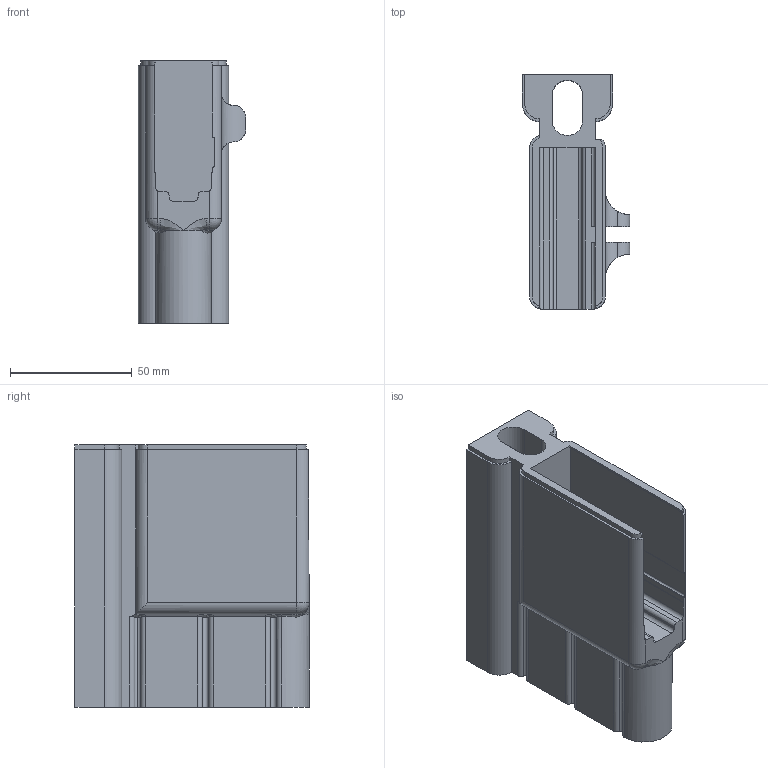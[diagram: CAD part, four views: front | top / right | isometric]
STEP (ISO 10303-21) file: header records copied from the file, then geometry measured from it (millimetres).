
FILE_DESCRIPTION (( 'STEP AP214' ), '1' );
FILE_NAME ('Charon_V3_Kommando_2.STEP', '2013-09-01T16:56:20', ( 'Asher' ), ( '' ), 'SwSTEP 2.0', 'SolidWorks 2013', '' );
FILE_SCHEMA (( 'AUTOMOTIVE_DESIGN' ));
Length unit declared in the file: millimetre
Products named in the file (1): Charon_V3_Kommando_2
Bounding box: 44.15 x 96.32 x 108 mm (x, y, z)
Volume: 154869.2 mm3; surface area: 53737.2 mm2
Topology: 1 solids, 1 shells, 219 faces, 628 edges, 402 vertices
Faces by surface type: cylinder 75, plane 69, sphere 32, cone 21, bspline 20, torus 2
Entity records: 9328 total; most frequent: CARTESIAN_POINT 3917, ORIENTED_EDGE 1140, DIRECTION 1100, EDGE_CURVE 570, AXIS2_PLACEMENT_3D 419, VERTEX_POINT 378, LINE 262, VECTOR 262
